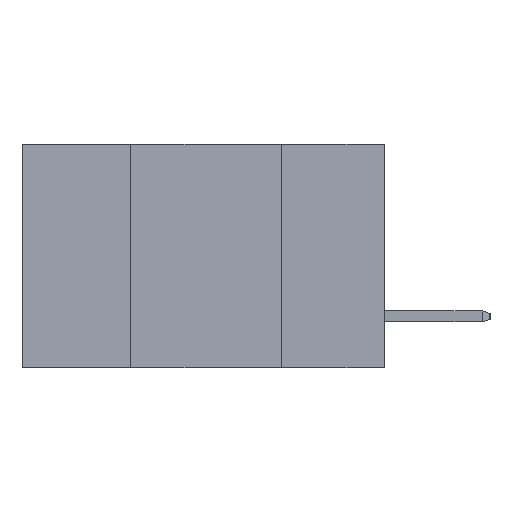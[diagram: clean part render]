
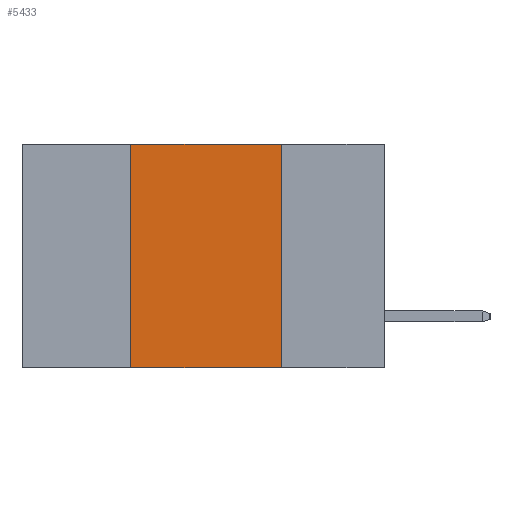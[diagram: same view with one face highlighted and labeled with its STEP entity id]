
A CAD part, left-side view. The second image highlights one B-rep face of the part: STEP entity #5433.
In plain terms, the highlighted planar face has unit normal (-1, 0, 0).
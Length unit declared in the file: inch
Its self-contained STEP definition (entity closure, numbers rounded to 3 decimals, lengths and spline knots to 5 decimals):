
#58 = VERTEX_POINT ( 'NONE', #901 ) ;
#163 = CARTESIAN_POINT ( 'NONE',  ( 0., 0.17, 0. ) ) ;
#901 = CARTESIAN_POINT ( 'NONE',  ( 0., 0.42, -0.37 ) ) ;
#1055 = CARTESIAN_POINT ( 'NONE',  ( 0., 0.6, 0. ) ) ;
#1214 = LINE ( 'NONE', #6758, #6289 ) ;
#2469 = PLANE ( 'NONE',  #11600 ) ;
#2486 = DIRECTION ( 'NONE',  ( 0., 0., -1. ) ) ;
#2945 = DIRECTION ( 'NONE',  ( 1., 0., 0. ) ) ;
#3881 = VERTEX_POINT ( 'NONE', #6924 ) ;
#4308 = ORIENTED_EDGE ( 'NONE', *, *, #10634, .F. ) ;
#4755 = CARTESIAN_POINT ( 'NONE',  ( 0., 0.17, 0. ) ) ;
#5433 = ADVANCED_FACE ( 'NONE', ( #6303 ), #2469, .F. ) ;
#5739 = EDGE_LOOP ( 'NONE', ( #4308, #11384, #6111, #11948 ) ) ;
#5805 = CARTESIAN_POINT ( 'NONE',  ( 0., 0.42, 0. ) ) ;
#6111 = ORIENTED_EDGE ( 'NONE', *, *, #10034, .F. ) ;
#6289 = VECTOR ( 'NONE', #10285, 39.37008 ) ;
#6303 = FACE_OUTER_BOUND ( 'NONE', #5739, .T. ) ;
#6758 = CARTESIAN_POINT ( 'NONE',  ( 0., 0.6, -0.37 ) ) ;
#6924 = CARTESIAN_POINT ( 'NONE',  ( 0., 0.17, -0.37 ) ) ;
#6996 = LINE ( 'NONE', #1055, #11459 ) ;
#6998 = CARTESIAN_POINT ( 'NONE',  ( 0., 0.6, 0. ) ) ;
#7023 = VECTOR ( 'NONE', #10395, 39.37008 ) ;
#7572 = LINE ( 'NONE', #5805, #7023 ) ;
#7977 = LINE ( 'NONE', #4755, #10368 ) ;
#9110 = CARTESIAN_POINT ( 'NONE',  ( 0., 0.42, 0. ) ) ;
#9423 = EDGE_CURVE ( 'NONE', #58, #3881, #1214, .T. ) ;
#9829 = DIRECTION ( 'NONE',  ( 0., -1., 0. ) ) ;
#10034 = EDGE_CURVE ( 'NONE', #58, #12247, #7572, .T. ) ;
#10285 = DIRECTION ( 'NONE',  ( 0., -1., 0. ) ) ;
#10340 = VERTEX_POINT ( 'NONE', #163 ) ;
#10368 = VECTOR ( 'NONE', #12086, 39.37008 ) ;
#10395 = DIRECTION ( 'NONE',  ( 0., 0., 1. ) ) ;
#10634 = EDGE_CURVE ( 'NONE', #10340, #3881, #7977, .T. ) ;
#10901 = EDGE_CURVE ( 'NONE', #12247, #10340, #6996, .T. ) ;
#11384 = ORIENTED_EDGE ( 'NONE', *, *, #10901, .F. ) ;
#11459 = VECTOR ( 'NONE', #9829, 39.37008 ) ;
#11600 = AXIS2_PLACEMENT_3D ( 'NONE', #6998, #2945, #2486 ) ;
#11948 = ORIENTED_EDGE ( 'NONE', *, *, #9423, .T. ) ;
#12086 = DIRECTION ( 'NONE',  ( 0., 0., -1. ) ) ;
#12247 = VERTEX_POINT ( 'NONE', #9110 ) ;
